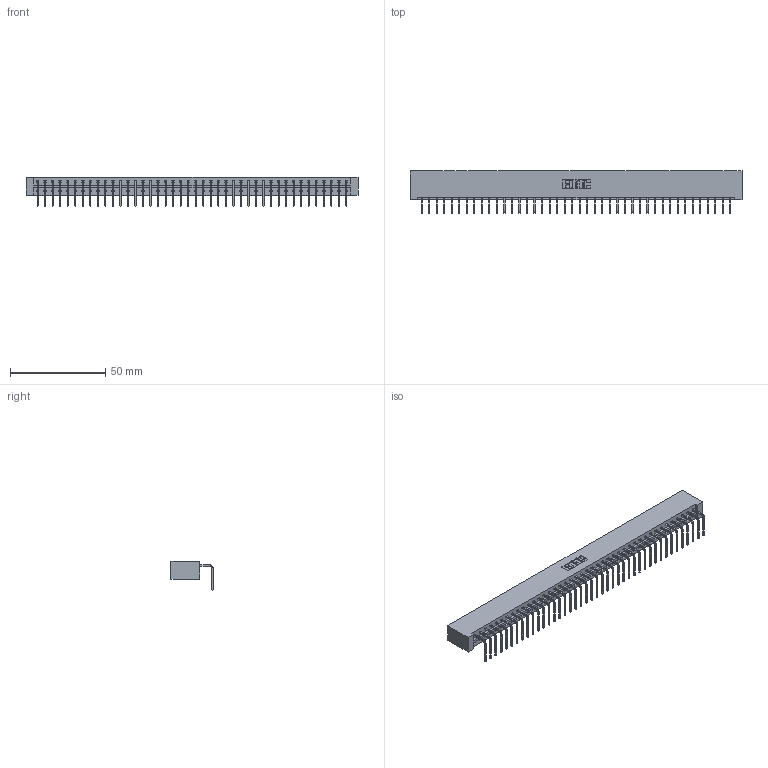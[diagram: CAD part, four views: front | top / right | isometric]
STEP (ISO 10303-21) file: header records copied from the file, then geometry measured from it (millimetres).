
FILE_DESCRIPTION (( 'STEP AP203' ), '1' );
FILE_NAME ('333-042-558-101.STEP', '2018-08-03T19:31:40', ( '' ), ( '' ), 'SwSTEP 2.0', 'SolidWorks 2016', '' );
FILE_SCHEMA (( 'CONFIG_CONTROL_DESIGN' ));
Length unit declared in the file: inch
Products named in the file (3): 345-292-001_558 Tail - 2; 333-042-558-101; 333 Part_Lugless
Assembly tree (43 placements, depth 2):
  333-042-558-101
    333 Part_Lugless
    345-292-001_558 Tail - 2  x42
Bounding box: 174.68 x 22.17 x 15.37 mm (x, y, z)
Volume: 18330 mm3; surface area: 20647.4 mm2
Topology: 43 solids, 43 shells, 2626 faces, 7931 edges, 5230 vertices
Faces by surface type: plane 1914, cylinder 712
Entity records: 25483 total; most frequent: CARTESIAN_POINT 4404, ORIENTED_EDGE 4382, DIRECTION 3707, EDGE_CURVE 2191, LINE 2071, VECTOR 2071, VERTEX_POINT 1458, AXIS2_PLACEMENT_3D 818
